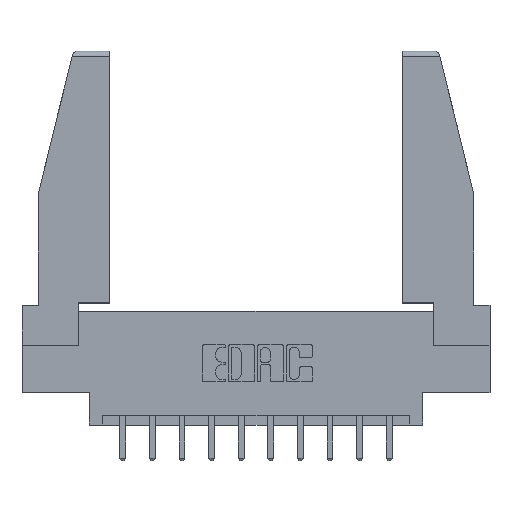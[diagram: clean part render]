
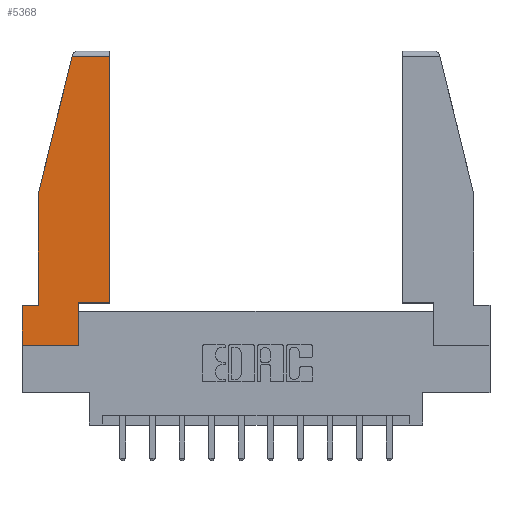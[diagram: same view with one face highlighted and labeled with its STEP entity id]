
A CAD part, top view. The second image highlights one B-rep face of the part: STEP entity #5368.
In plain terms, the highlighted planar face has unit normal (0, 0, 1).
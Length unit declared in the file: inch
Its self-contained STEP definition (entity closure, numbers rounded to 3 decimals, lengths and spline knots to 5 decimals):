
#53 = VERTEX_POINT ( 'NONE', #2384 ) ;
#69 = CARTESIAN_POINT ( 'NONE',  ( 0., 0., 0. ) ) ;
#522 = CARTESIAN_POINT ( 'NONE',  ( 0., 0.21, 0. ) ) ;
#732 = ORIENTED_EDGE ( 'NONE', *, *, #5035, .T. ) ;
#856 = VERTEX_POINT ( 'NONE', #11122 ) ;
#1164 = VECTOR ( 'NONE', #7970, 39.37008 ) ;
#1209 = EDGE_CURVE ( 'NONE', #13377, #2478, #5037, .T. ) ;
#1299 = DIRECTION ( 'NONE',  ( 1., 0., 0. ) ) ;
#1423 = LINE ( 'NONE', #69, #7880 ) ;
#1572 = ORIENTED_EDGE ( 'NONE', *, *, #10461, .T. ) ;
#1969 = DIRECTION ( 'NONE',  ( -1., 0., 0. ) ) ;
#2067 = VECTOR ( 'NONE', #9576, 39.37008 ) ;
#2254 = ORIENTED_EDGE ( 'NONE', *, *, #6866, .T. ) ;
#2384 = CARTESIAN_POINT ( 'NONE',  ( 0.2636, 1.52, 0. ) ) ;
#2478 = VERTEX_POINT ( 'NONE', #5267 ) ;
#2563 = AXIS2_PLACEMENT_3D ( 'NONE', #5049, #11898, #6192 ) ;
#2785 = EDGE_CURVE ( 'NONE', #856, #7685, #14012, .T. ) ;
#2839 = EDGE_CURVE ( 'NONE', #9013, #13377, #4494, .T. ) ;
#3347 = ORIENTED_EDGE ( 'NONE', *, *, #8398, .T. ) ;
#3798 = VECTOR ( 'NONE', #10509, 39.37008 ) ;
#3899 = PLANE ( 'NONE',  #2563 ) ;
#4067 = CARTESIAN_POINT ( 'NONE',  ( 0., 0.21, 0. ) ) ;
#4401 = EDGE_CURVE ( 'NONE', #7685, #10927, #9026, .T. ) ;
#4494 = LINE ( 'NONE', #6170, #11165 ) ;
#4572 = ORIENTED_EDGE ( 'NONE', *, *, #4401, .T. ) ;
#4941 = CARTESIAN_POINT ( 'NONE',  ( 0.461, 1.52, 0. ) ) ;
#5035 = EDGE_CURVE ( 'NONE', #2478, #10314, #7913, .T. ) ;
#5037 = LINE ( 'NONE', #522, #2067 ) ;
#5049 = CARTESIAN_POINT ( 'NONE',  ( 0., 0., 0. ) ) ;
#5267 = CARTESIAN_POINT ( 'NONE',  ( 0., 0.21, 0. ) ) ;
#5368 = ADVANCED_FACE ( 'NONE', ( #5641 ), #3899, .T. ) ;
#5641 = FACE_OUTER_BOUND ( 'NONE', #10184, .T. ) ;
#5718 = ORIENTED_EDGE ( 'NONE', *, *, #2839, .T. ) ;
#5921 = ORIENTED_EDGE ( 'NONE', *, *, #1209, .T. ) ;
#5931 = CARTESIAN_POINT ( 'NONE',  ( 0.297, 0., 0. ) ) ;
#6170 = CARTESIAN_POINT ( 'NONE',  ( 0.086, 0.8, 0. ) ) ;
#6192 = DIRECTION ( 'NONE',  ( 1., 0., 0. ) ) ;
#6267 = DIRECTION ( 'NONE',  ( 0., -1., 0. ) ) ;
#6639 = CARTESIAN_POINT ( 'NONE',  ( 0., 0., 0. ) ) ;
#6866 = EDGE_CURVE ( 'NONE', #53, #9013, #11890, .T. ) ;
#7041 = LINE ( 'NONE', #13337, #11118 ) ;
#7593 = CARTESIAN_POINT ( 'NONE',  ( 0., 1.52, 0. ) ) ;
#7682 = CARTESIAN_POINT ( 'NONE',  ( 0.461, 0.223, 0. ) ) ;
#7685 = VERTEX_POINT ( 'NONE', #11603 ) ;
#7880 = VECTOR ( 'NONE', #9081, 39.37008 ) ;
#7913 = LINE ( 'NONE', #4067, #8275 ) ;
#7970 = DIRECTION ( 'NONE',  ( -0.239, -0.971, 0. ) ) ;
#8275 = VECTOR ( 'NONE', #6267, 39.37008 ) ;
#8398 = EDGE_CURVE ( 'NONE', #10927, #13778, #7041, .T. ) ;
#8601 = CARTESIAN_POINT ( 'NONE',  ( 0.086, 0.21, 0. ) ) ;
#8699 = ORIENTED_EDGE ( 'NONE', *, *, #13392, .T. ) ;
#8855 = DIRECTION ( 'NONE',  ( 0., 1., 0. ) ) ;
#9013 = VERTEX_POINT ( 'NONE', #9751 ) ;
#9026 = LINE ( 'NONE', #12383, #13797 ) ;
#9081 = DIRECTION ( 'NONE',  ( 1., 0., 0. ) ) ;
#9441 = LINE ( 'NONE', #7593, #12226 ) ;
#9576 = DIRECTION ( 'NONE',  ( -1., 0., 0. ) ) ;
#9751 = CARTESIAN_POINT ( 'NONE',  ( 0.086, 0.8, 0. ) ) ;
#10184 = EDGE_LOOP ( 'NONE', ( #3347, #8699, #2254, #5718, #5921, #732, #1572, #14030, #4572 ) ) ;
#10314 = VERTEX_POINT ( 'NONE', #6639 ) ;
#10461 = EDGE_CURVE ( 'NONE', #10314, #856, #1423, .T. ) ;
#10509 = DIRECTION ( 'NONE',  ( 0., 1., 0. ) ) ;
#10927 = VERTEX_POINT ( 'NONE', #7682 ) ;
#11118 = VECTOR ( 'NONE', #8855, 39.37008 ) ;
#11122 = CARTESIAN_POINT ( 'NONE',  ( 0.297, 0., 0. ) ) ;
#11165 = VECTOR ( 'NONE', #11729, 39.37008 ) ;
#11603 = CARTESIAN_POINT ( 'NONE',  ( 0.297, 0.223, 0. ) ) ;
#11729 = DIRECTION ( 'NONE',  ( 0., -1., 0. ) ) ;
#11890 = LINE ( 'NONE', #13542, #1164 ) ;
#11898 = DIRECTION ( 'NONE',  ( 0., 0., 1. ) ) ;
#12226 = VECTOR ( 'NONE', #1969, 39.37008 ) ;
#12383 = CARTESIAN_POINT ( 'NONE',  ( 0.297, 0.223, 0. ) ) ;
#13337 = CARTESIAN_POINT ( 'NONE',  ( 0.461, 0.223, 0. ) ) ;
#13377 = VERTEX_POINT ( 'NONE', #8601 ) ;
#13392 = EDGE_CURVE ( 'NONE', #13778, #53, #9441, .T. ) ;
#13542 = CARTESIAN_POINT ( 'NONE',  ( 0.271, 1.55, 0. ) ) ;
#13778 = VERTEX_POINT ( 'NONE', #4941 ) ;
#13797 = VECTOR ( 'NONE', #1299, 39.37008 ) ;
#14012 = LINE ( 'NONE', #5931, #3798 ) ;
#14030 = ORIENTED_EDGE ( 'NONE', *, *, #2785, .T. ) ;
